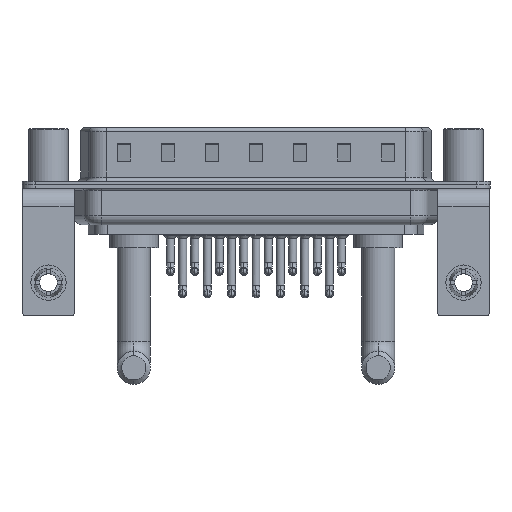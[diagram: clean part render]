
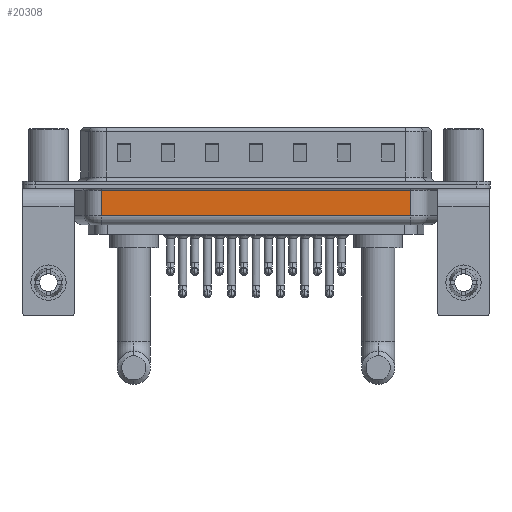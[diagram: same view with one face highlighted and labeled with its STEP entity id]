
A CAD part, front view. The second image highlights one B-rep face of the part: STEP entity #20308.
In plain terms, the highlighted planar face has unit normal (0, -1, 0).
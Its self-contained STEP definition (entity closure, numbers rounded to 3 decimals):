
#1679 = VERTEX_POINT ( 'NONE', #1760 ) ;
#1760 = CARTESIAN_POINT ( 'NONE',  ( 6.006, -5.35, -0.65 ) ) ;
#2030 = CARTESIAN_POINT ( 'NONE',  ( 6.006, -5.35, -4.5 ) ) ;
#2094 = CARTESIAN_POINT ( 'NONE',  ( 6.006, -5.35, -3.5 ) ) ;
#2908 = EDGE_CURVE ( 'NONE', #21414, #14144, #20547, .T. ) ;
#3217 = CARTESIAN_POINT ( 'NONE',  ( 6.006, -5.35, -4.5 ) ) ;
#3626 = ORIENTED_EDGE ( 'NONE', *, *, #3849, .T. ) ;
#3849 = EDGE_CURVE ( 'NONE', #9405, #21414, #18456, .T. ) ;
#6808 = CARTESIAN_POINT ( 'NONE',  ( 41.044, -5.35, -4.5 ) ) ;
#7092 = DIRECTION ( 'NONE',  ( 0., 0., 1. ) ) ;
#7448 = AXIS2_PLACEMENT_3D ( 'NONE', #3217, #16144, #18739 ) ;
#9188 = EDGE_CURVE ( 'NONE', #14144, #1679, #28756, .T. ) ;
#9405 = VERTEX_POINT ( 'NONE', #2094 ) ;
#11381 = DIRECTION ( 'NONE',  ( -1., 0., 0. ) ) ;
#13142 = ORIENTED_EDGE ( 'NONE', *, *, #23079, .F. ) ;
#14144 = VERTEX_POINT ( 'NONE', #14775 ) ;
#14775 = CARTESIAN_POINT ( 'NONE',  ( 41.044, -5.35, -0.65 ) ) ;
#16144 = DIRECTION ( 'NONE',  ( 0., 1., 0. ) ) ;
#18288 = CARTESIAN_POINT ( 'NONE',  ( 41.044, -5.35, -3.5 ) ) ;
#18456 = LINE ( 'NONE', #22817, #19257 ) ;
#18739 = DIRECTION ( 'NONE',  ( 0., 0., 1. ) ) ;
#19257 = VECTOR ( 'NONE', #27046, 1000. ) ;
#19854 = CARTESIAN_POINT ( 'NONE',  ( 6.006, -5.35, -0.65 ) ) ;
#19900 = EDGE_LOOP ( 'NONE', ( #13142, #3626, #23898, #20010 ) ) ;
#20010 = ORIENTED_EDGE ( 'NONE', *, *, #9188, .T. ) ;
#20131 = DIRECTION ( 'NONE',  ( 0., 0., 1. ) ) ;
#20308 = ADVANCED_FACE ( 'NONE', ( #25301 ), #22824, .F. ) ;
#20547 = LINE ( 'NONE', #6808, #20610 ) ;
#20610 = VECTOR ( 'NONE', #7092, 1000. ) ;
#21414 = VERTEX_POINT ( 'NONE', #18288 ) ;
#22044 = LINE ( 'NONE', #2030, #27172 ) ;
#22817 = CARTESIAN_POINT ( 'NONE',  ( 6.006, -5.35, -3.5 ) ) ;
#22824 = PLANE ( 'NONE',  #7448 ) ;
#23079 = EDGE_CURVE ( 'NONE', #9405, #1679, #22044, .T. ) ;
#23898 = ORIENTED_EDGE ( 'NONE', *, *, #2908, .T. ) ;
#24622 = VECTOR ( 'NONE', #11381, 1000. ) ;
#25301 = FACE_OUTER_BOUND ( 'NONE', #19900, .T. ) ;
#27046 = DIRECTION ( 'NONE',  ( 1., 0., 0. ) ) ;
#27172 = VECTOR ( 'NONE', #20131, 1000. ) ;
#28756 = LINE ( 'NONE', #19854, #24622 ) ;
